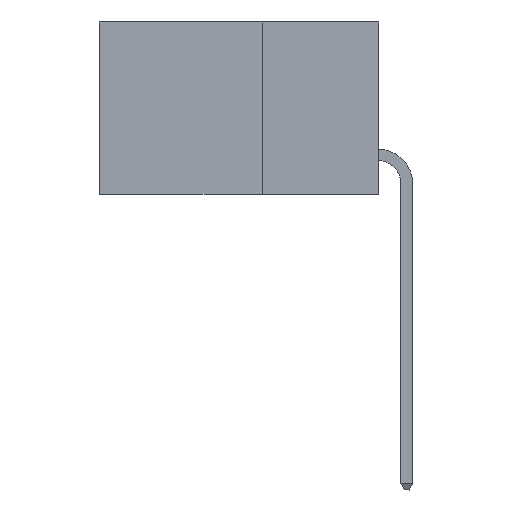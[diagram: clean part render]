
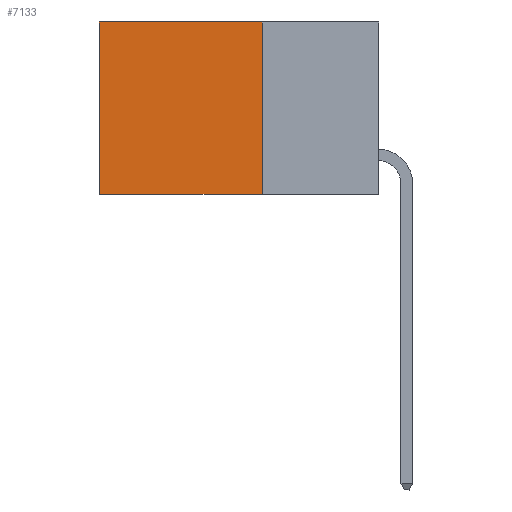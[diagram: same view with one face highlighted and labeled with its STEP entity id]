
A CAD part, left-side view. The second image highlights one B-rep face of the part: STEP entity #7133.
In plain terms, the highlighted planar face has unit normal (-1, 0, 0).
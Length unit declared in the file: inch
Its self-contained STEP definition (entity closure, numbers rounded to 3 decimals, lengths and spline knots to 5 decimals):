
#563 = EDGE_CURVE ( 'NONE', #11440, #675, #8896, .T. ) ;
#675 = VERTEX_POINT ( 'NONE', #10255 ) ;
#1333 = DIRECTION ( 'NONE',  ( 0., 0., -1. ) ) ;
#1648 = EDGE_CURVE ( 'NONE', #11440, #3136, #5504, .T. ) ;
#1997 = CARTESIAN_POINT ( 'NONE',  ( 0.2615, 0.25, -0.37 ) ) ;
#2730 = CARTESIAN_POINT ( 'NONE',  ( 0.2615, 0.6, 0. ) ) ;
#2925 = DIRECTION ( 'NONE',  ( 0., 0., -1. ) ) ;
#3009 = CARTESIAN_POINT ( 'NONE',  ( 0.2615, 0.6, -0.37 ) ) ;
#3136 = VERTEX_POINT ( 'NONE', #2730 ) ;
#3346 = EDGE_CURVE ( 'NONE', #3136, #9666, #12231, .T. ) ;
#3852 = ORIENTED_EDGE ( 'NONE', *, *, #563, .F. ) ;
#4017 = VECTOR ( 'NONE', #2925, 39.37008 ) ;
#4287 = CARTESIAN_POINT ( 'NONE',  ( 0.2615, 0.6, -0.37 ) ) ;
#4291 = VECTOR ( 'NONE', #8327, 39.37008 ) ;
#4326 = LINE ( 'NONE', #4455, #4291 ) ;
#4455 = CARTESIAN_POINT ( 'NONE',  ( 0.2615, 0.25, -0.37 ) ) ;
#5277 = DIRECTION ( 'NONE',  ( 0., 0., -1. ) ) ;
#5504 = LINE ( 'NONE', #10555, #10318 ) ;
#5529 = EDGE_CURVE ( 'NONE', #675, #9666, #4326, .T. ) ;
#6005 = ORIENTED_EDGE ( 'NONE', *, *, #3346, .T. ) ;
#6404 = PLANE ( 'NONE',  #7675 ) ;
#6513 = ORIENTED_EDGE ( 'NONE', *, *, #5529, .F. ) ;
#6600 = CARTESIAN_POINT ( 'NONE',  ( 0.2615, 0.25, -0.37 ) ) ;
#6719 = EDGE_LOOP ( 'NONE', ( #6005, #6513, #3852, #7457 ) ) ;
#7133 = ADVANCED_FACE ( 'NONE', ( #10526 ), #6404, .F. ) ;
#7359 = CARTESIAN_POINT ( 'NONE',  ( 0.2615, 0.25, 0. ) ) ;
#7417 = DIRECTION ( 'NONE',  ( 0., 1., 0. ) ) ;
#7457 = ORIENTED_EDGE ( 'NONE', *, *, #1648, .T. ) ;
#7521 = DIRECTION ( 'NONE',  ( 1., 0., 0. ) ) ;
#7675 = AXIS2_PLACEMENT_3D ( 'NONE', #6600, #7521, #5277 ) ;
#8062 = VECTOR ( 'NONE', #1333, 39.37008 ) ;
#8327 = DIRECTION ( 'NONE',  ( 0., 1., 0. ) ) ;
#8896 = LINE ( 'NONE', #1997, #4017 ) ;
#9666 = VERTEX_POINT ( 'NONE', #3009 ) ;
#10255 = CARTESIAN_POINT ( 'NONE',  ( 0.2615, 0.25, -0.37 ) ) ;
#10318 = VECTOR ( 'NONE', #7417, 39.37008 ) ;
#10526 = FACE_OUTER_BOUND ( 'NONE', #6719, .T. ) ;
#10555 = CARTESIAN_POINT ( 'NONE',  ( 0.2615, 0.25, 0. ) ) ;
#11440 = VERTEX_POINT ( 'NONE', #7359 ) ;
#12231 = LINE ( 'NONE', #4287, #8062 ) ;
